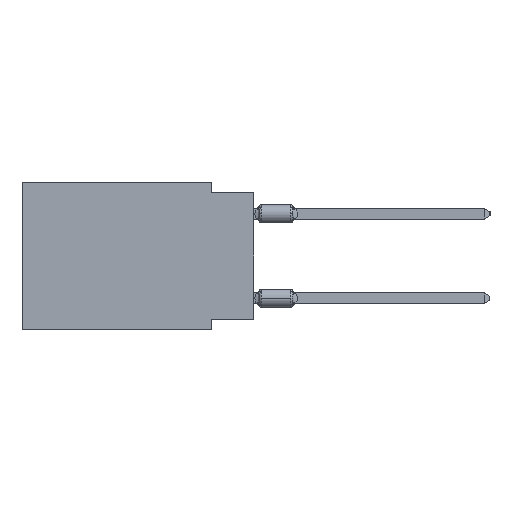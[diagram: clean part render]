
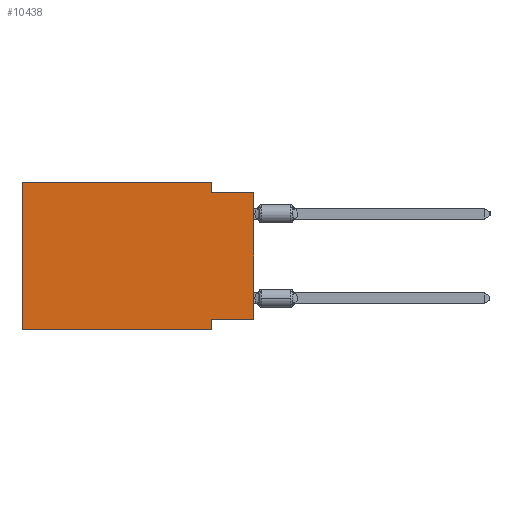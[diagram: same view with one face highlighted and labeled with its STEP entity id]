
A CAD part, left-side view. The second image highlights one B-rep face of the part: STEP entity #10438.
In plain terms, the highlighted planar face has unit normal (-1, 0, 0).
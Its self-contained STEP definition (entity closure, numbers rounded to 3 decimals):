
#2551 = DIRECTION ( 'NONE',  ( 0., 1., 0. ) ) ;
#3083 = EDGE_CURVE ( 'NONE', #50144, #20148, #23903, .T. ) ;
#7112 = ORIENTED_EDGE ( 'NONE', *, *, #3083, .T. ) ;
#7781 = EDGE_CURVE ( 'NONE', #28235, #62180, #36618, .T. ) ;
#7798 = FACE_OUTER_BOUND ( 'NONE', #24362, .T. ) ;
#8407 = VECTOR ( 'NONE', #22167, 1000. ) ;
#10438 = ADVANCED_FACE ( 'NONE', ( #7798 ), #21763, .F. ) ;
#11954 = DIRECTION ( 'NONE',  ( 0., -1., 0. ) ) ;
#12695 = CARTESIAN_POINT ( 'NONE',  ( 0., 0., -0.635 ) ) ;
#14392 = CARTESIAN_POINT ( 'NONE',  ( 0., 2.54, -8.255 ) ) ;
#15300 = CARTESIAN_POINT ( 'NONE',  ( 0., 0., -8.255 ) ) ;
#16685 = CARTESIAN_POINT ( 'NONE',  ( 0., 2.54, -8.89 ) ) ;
#17224 = EDGE_CURVE ( 'NONE', #32066, #62180, #52107, .T. ) ;
#17528 = DIRECTION ( 'NONE',  ( 1., 0., 0. ) ) ;
#17565 = DIRECTION ( 'NONE',  ( 0., 0., 1. ) ) ;
#18061 = VECTOR ( 'NONE', #40055, 1000. ) ;
#18617 = LINE ( 'NONE', #37764, #60834 ) ;
#18787 = CARTESIAN_POINT ( 'NONE',  ( 0., 13.97, -8.89 ) ) ;
#20148 = VERTEX_POINT ( 'NONE', #12695 ) ;
#20623 = EDGE_CURVE ( 'NONE', #50144, #32066, #47005, .T. ) ;
#21468 = EDGE_CURVE ( 'NONE', #28235, #32267, #48071, .T. ) ;
#21763 = PLANE ( 'NONE',  #63290 ) ;
#21846 = LINE ( 'NONE', #55281, #8407 ) ;
#22167 = DIRECTION ( 'NONE',  ( 0., -1., 0. ) ) ;
#22262 = CARTESIAN_POINT ( 'NONE',  ( 0., 2.54, -8.89 ) ) ;
#22821 = VECTOR ( 'NONE', #2551, 1000. ) ;
#23067 = DIRECTION ( 'NONE',  ( 0., 0., -1. ) ) ;
#23802 = ORIENTED_EDGE ( 'NONE', *, *, #20623, .F. ) ;
#23903 = LINE ( 'NONE', #34560, #18061 ) ;
#24362 = EDGE_LOOP ( 'NONE', ( #7112, #42132, #60893, #47194, #36700, #37598, #27811, #23802 ) ) ;
#27185 = CARTESIAN_POINT ( 'NONE',  ( 0., 2.54, 0. ) ) ;
#27811 = ORIENTED_EDGE ( 'NONE', *, *, #17224, .F. ) ;
#28235 = VERTEX_POINT ( 'NONE', #18787 ) ;
#28721 = VECTOR ( 'NONE', #38142, 1000. ) ;
#29030 = EDGE_CURVE ( 'NONE', #32267, #62659, #18617, .T. ) ;
#32066 = VERTEX_POINT ( 'NONE', #14392 ) ;
#32267 = VERTEX_POINT ( 'NONE', #35135 ) ;
#34238 = EDGE_CURVE ( 'NONE', #62659, #37591, #57385, .T. ) ;
#34560 = CARTESIAN_POINT ( 'NONE',  ( 0., 0., 0. ) ) ;
#35135 = CARTESIAN_POINT ( 'NONE',  ( 0., 13.97, 0. ) ) ;
#36618 = LINE ( 'NONE', #52513, #49713 ) ;
#36700 = ORIENTED_EDGE ( 'NONE', *, *, #21468, .F. ) ;
#37591 = VERTEX_POINT ( 'NONE', #51953 ) ;
#37598 = ORIENTED_EDGE ( 'NONE', *, *, #7781, .T. ) ;
#37764 = CARTESIAN_POINT ( 'NONE',  ( 0., 13.97, 0. ) ) ;
#38142 = DIRECTION ( 'NONE',  ( 0., 0., -1. ) ) ;
#40055 = DIRECTION ( 'NONE',  ( 0., 0., 1. ) ) ;
#42132 = ORIENTED_EDGE ( 'NONE', *, *, #46491, .F. ) ;
#46491 = EDGE_CURVE ( 'NONE', #37591, #20148, #21846, .T. ) ;
#47005 = LINE ( 'NONE', #51881, #22821 ) ;
#47194 = ORIENTED_EDGE ( 'NONE', *, *, #29030, .F. ) ;
#48071 = LINE ( 'NONE', #63307, #51725 ) ;
#49713 = VECTOR ( 'NONE', #11954, 1000. ) ;
#50144 = VERTEX_POINT ( 'NONE', #15300 ) ;
#51725 = VECTOR ( 'NONE', #17565, 1000. ) ;
#51881 = CARTESIAN_POINT ( 'NONE',  ( 0., 0., -8.255 ) ) ;
#51953 = CARTESIAN_POINT ( 'NONE',  ( 0., 2.54, -0.635 ) ) ;
#52107 = LINE ( 'NONE', #22262, #28721 ) ;
#52258 = CARTESIAN_POINT ( 'NONE',  ( 0., 13.97, 0. ) ) ;
#52513 = CARTESIAN_POINT ( 'NONE',  ( 0., 13.97, -8.89 ) ) ;
#53656 = DIRECTION ( 'NONE',  ( 0., -1., 0. ) ) ;
#54075 = VECTOR ( 'NONE', #57703, 1000. ) ;
#55281 = CARTESIAN_POINT ( 'NONE',  ( 0., 0., -0.635 ) ) ;
#57385 = LINE ( 'NONE', #27185, #54075 ) ;
#57703 = DIRECTION ( 'NONE',  ( 0., 0., -1. ) ) ;
#60834 = VECTOR ( 'NONE', #53656, 1000. ) ;
#60893 = ORIENTED_EDGE ( 'NONE', *, *, #34238, .F. ) ;
#62180 = VERTEX_POINT ( 'NONE', #16685 ) ;
#62613 = CARTESIAN_POINT ( 'NONE',  ( 0., 2.54, 0. ) ) ;
#62659 = VERTEX_POINT ( 'NONE', #62613 ) ;
#63290 = AXIS2_PLACEMENT_3D ( 'NONE', #52258, #17528, #23067 ) ;
#63307 = CARTESIAN_POINT ( 'NONE',  ( 0., 13.97, 0. ) ) ;
